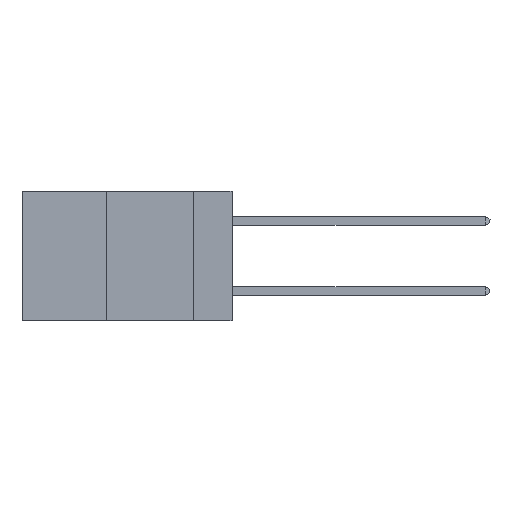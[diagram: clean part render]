
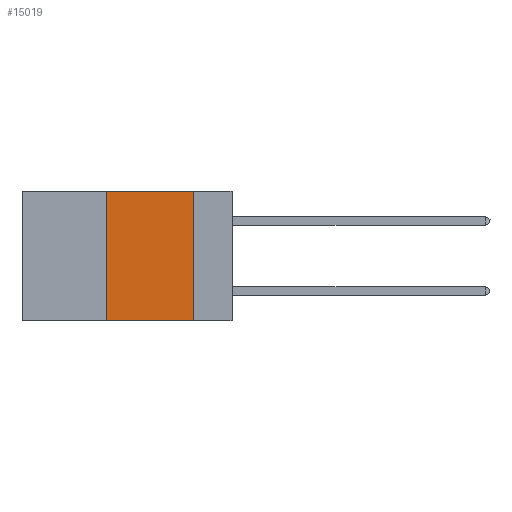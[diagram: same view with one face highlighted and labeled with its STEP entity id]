
A CAD part, left-side view. The second image highlights one B-rep face of the part: STEP entity #15019.
In plain terms, the highlighted planar face has unit normal (-1, 0, 0).
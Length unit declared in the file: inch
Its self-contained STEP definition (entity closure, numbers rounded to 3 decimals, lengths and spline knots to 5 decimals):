
#2644 = LINE ( 'NONE', #21176, #15566 ) ;
#2953 = EDGE_CURVE ( 'NONE', #43359, #9496, #14071, .T. ) ;
#3259 = CARTESIAN_POINT ( 'NONE',  ( 0., 0.11, 0. ) ) ;
#4151 = EDGE_CURVE ( 'NONE', #15530, #14076, #2644, .T. ) ;
#4216 = DIRECTION ( 'NONE',  ( 1., 0., 0. ) ) ;
#4726 = DIRECTION ( 'NONE',  ( 0., -1., 0. ) ) ;
#4776 = EDGE_CURVE ( 'NONE', #43359, #14076, #36447, .T. ) ;
#5324 = CARTESIAN_POINT ( 'NONE',  ( 0., 0.6, -0.37 ) ) ;
#6227 = CARTESIAN_POINT ( 'NONE',  ( 0., 0.6, 0. ) ) ;
#9496 = VERTEX_POINT ( 'NONE', #30078 ) ;
#10705 = CARTESIAN_POINT ( 'NONE',  ( 0., 0.36, 0. ) ) ;
#10853 = DIRECTION ( 'NONE',  ( 0., 0., -1. ) ) ;
#14071 = LINE ( 'NONE', #10705, #25338 ) ;
#14076 = VERTEX_POINT ( 'NONE', #39463 ) ;
#14151 = DIRECTION ( 'NONE',  ( 0., 0., -1. ) ) ;
#14762 = PLANE ( 'NONE',  #19435 ) ;
#15019 = ADVANCED_FACE ( 'NONE', ( #42607 ), #14762, .F. ) ;
#15150 = VECTOR ( 'NONE', #41365, 39.37008 ) ;
#15530 = VERTEX_POINT ( 'NONE', #3259 ) ;
#15566 = VECTOR ( 'NONE', #14151, 39.37008 ) ;
#16766 = LINE ( 'NONE', #6227, #15150 ) ;
#16997 = DIRECTION ( 'NONE',  ( 0., 0., 1. ) ) ;
#18197 = CARTESIAN_POINT ( 'NONE',  ( 0., 0.6, 0. ) ) ;
#19435 = AXIS2_PLACEMENT_3D ( 'NONE', #18197, #4216, #10853 ) ;
#20535 = ORIENTED_EDGE ( 'NONE', *, *, #2953, .F. ) ;
#21176 = CARTESIAN_POINT ( 'NONE',  ( 0., 0.11, 0. ) ) ;
#25148 = ORIENTED_EDGE ( 'NONE', *, *, #4151, .F. ) ;
#25338 = VECTOR ( 'NONE', #16997, 39.37008 ) ;
#25404 = ORIENTED_EDGE ( 'NONE', *, *, #27737, .F. ) ;
#27737 = EDGE_CURVE ( 'NONE', #9496, #15530, #16766, .T. ) ;
#30078 = CARTESIAN_POINT ( 'NONE',  ( 0., 0.36, 0. ) ) ;
#36447 = LINE ( 'NONE', #5324, #39157 ) ;
#38838 = EDGE_LOOP ( 'NONE', ( #25148, #25404, #20535, #39312 ) ) ;
#39157 = VECTOR ( 'NONE', #4726, 39.37008 ) ;
#39312 = ORIENTED_EDGE ( 'NONE', *, *, #4776, .T. ) ;
#39463 = CARTESIAN_POINT ( 'NONE',  ( 0., 0.11, -0.37 ) ) ;
#40279 = CARTESIAN_POINT ( 'NONE',  ( 0., 0.36, -0.37 ) ) ;
#41365 = DIRECTION ( 'NONE',  ( 0., -1., 0. ) ) ;
#42607 = FACE_OUTER_BOUND ( 'NONE', #38838, .T. ) ;
#43359 = VERTEX_POINT ( 'NONE', #40279 ) ;
